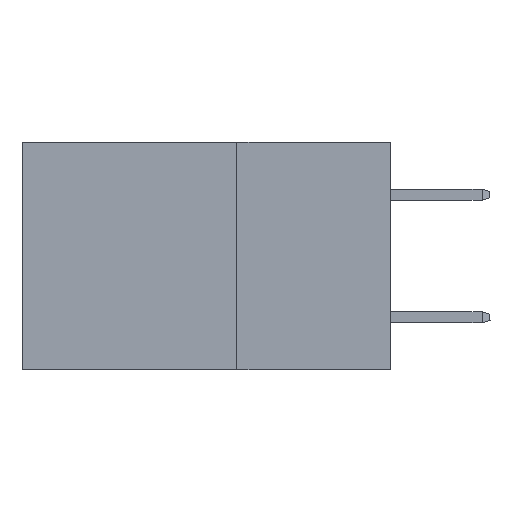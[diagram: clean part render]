
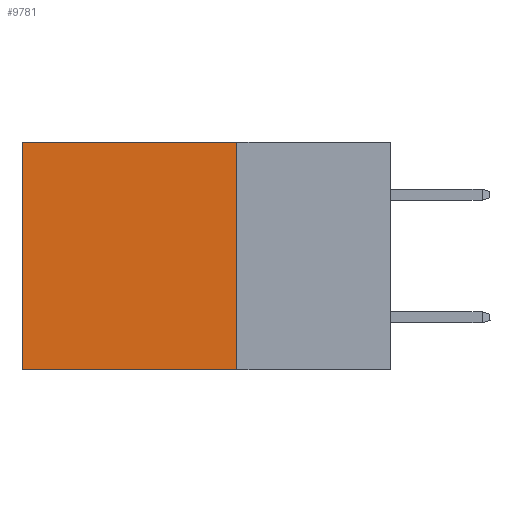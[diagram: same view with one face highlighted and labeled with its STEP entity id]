
A CAD part, left-side view. The second image highlights one B-rep face of the part: STEP entity #9781.
In plain terms, the highlighted planar face has unit normal (-1, 0, 0).
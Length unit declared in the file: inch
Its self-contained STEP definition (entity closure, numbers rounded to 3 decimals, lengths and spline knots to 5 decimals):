
#346 = FACE_OUTER_BOUND ( 'NONE', #11404, .T. ) ;
#550 = VERTEX_POINT ( 'NONE', #17480 ) ;
#964 = DIRECTION ( 'NONE',  ( 0., 0., -1. ) ) ;
#1271 = CARTESIAN_POINT ( 'NONE',  ( 0.2875, 0.25, 0. ) ) ;
#2739 = DIRECTION ( 'NONE',  ( 0., 1., 0. ) ) ;
#2965 = PLANE ( 'NONE',  #13235 ) ;
#3052 = ORIENTED_EDGE ( 'NONE', *, *, #4597, .T. ) ;
#3906 = EDGE_CURVE ( 'NONE', #7409, #7158, #7789, .T. ) ;
#3972 = ORIENTED_EDGE ( 'NONE', *, *, #13833, .F. ) ;
#4597 = EDGE_CURVE ( 'NONE', #550, #7158, #6437, .T. ) ;
#4713 = DIRECTION ( 'NONE',  ( 1., 0., 0. ) ) ;
#4775 = CARTESIAN_POINT ( 'NONE',  ( 0.2875, 0.6, -0.37 ) ) ;
#4941 = CARTESIAN_POINT ( 'NONE',  ( 0.2875, 0.25, 0. ) ) ;
#5432 = CARTESIAN_POINT ( 'NONE',  ( 0.2875, 0.6, 0. ) ) ;
#5891 = VECTOR ( 'NONE', #7635, 39.37008 ) ;
#6437 = LINE ( 'NONE', #5432, #5891 ) ;
#7119 = CARTESIAN_POINT ( 'NONE',  ( 0.2875, 0.25, -0.37 ) ) ;
#7158 = VERTEX_POINT ( 'NONE', #4775 ) ;
#7409 = VERTEX_POINT ( 'NONE', #7119 ) ;
#7635 = DIRECTION ( 'NONE',  ( 0., 0., -1. ) ) ;
#7789 = LINE ( 'NONE', #9479, #11805 ) ;
#7914 = VECTOR ( 'NONE', #964, 39.37008 ) ;
#9479 = CARTESIAN_POINT ( 'NONE',  ( 0.2875, 0.25, -0.37 ) ) ;
#9781 = ADVANCED_FACE ( 'NONE', ( #346 ), #2965, .F. ) ;
#11022 = VERTEX_POINT ( 'NONE', #11293 ) ;
#11293 = CARTESIAN_POINT ( 'NONE',  ( 0.2875, 0.25, 0. ) ) ;
#11404 = EDGE_LOOP ( 'NONE', ( #3052, #18448, #3972, #16205 ) ) ;
#11805 = VECTOR ( 'NONE', #2739, 39.37008 ) ;
#11860 = VECTOR ( 'NONE', #16775, 39.37008 ) ;
#13235 = AXIS2_PLACEMENT_3D ( 'NONE', #1271, #4713, #16570 ) ;
#13833 = EDGE_CURVE ( 'NONE', #11022, #7409, #21311, .T. ) ;
#15625 = EDGE_CURVE ( 'NONE', #11022, #550, #20241, .T. ) ;
#16205 = ORIENTED_EDGE ( 'NONE', *, *, #15625, .T. ) ;
#16570 = DIRECTION ( 'NONE',  ( 0., 0., -1. ) ) ;
#16775 = DIRECTION ( 'NONE',  ( 0., 1., 0. ) ) ;
#17480 = CARTESIAN_POINT ( 'NONE',  ( 0.2875, 0.6, 0. ) ) ;
#18448 = ORIENTED_EDGE ( 'NONE', *, *, #3906, .F. ) ;
#20241 = LINE ( 'NONE', #4941, #11860 ) ;
#21186 = CARTESIAN_POINT ( 'NONE',  ( 0.2875, 0.25, 0. ) ) ;
#21311 = LINE ( 'NONE', #21186, #7914 ) ;
